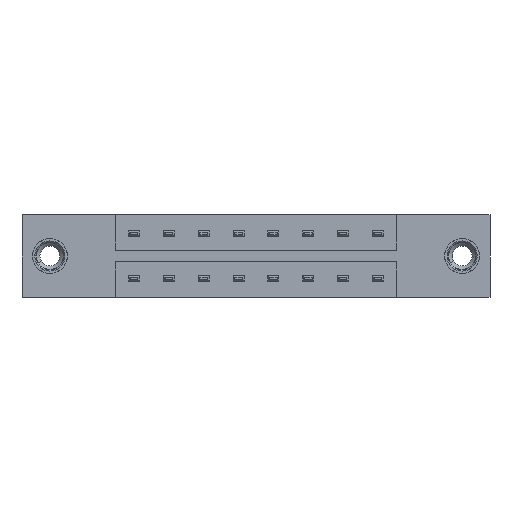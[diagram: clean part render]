
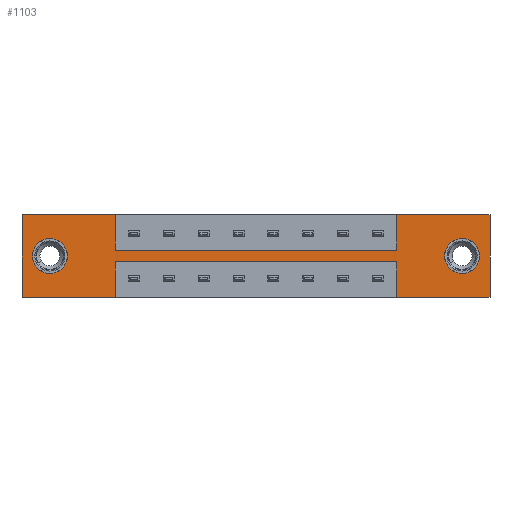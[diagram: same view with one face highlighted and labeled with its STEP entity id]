
A CAD part, front view. The second image highlights one B-rep face of the part: STEP entity #1103.
In plain terms, the highlighted planar face has unit normal (0, -1, 0).
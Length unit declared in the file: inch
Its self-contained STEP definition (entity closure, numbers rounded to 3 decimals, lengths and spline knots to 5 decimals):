
#28 = CARTESIAN_POINT ( 'NONE',  ( 0.125, 0., -0.107 ) ) ;
#279 = CIRCLE ( 'NONE', #1157, 0.078 ) ;
#281 = VERTEX_POINT ( 'NONE', #5145 ) ;
#287 = CARTESIAN_POINT ( 'NONE',  ( 1.6785, 0., -0.2115 ) ) ;
#428 = CARTESIAN_POINT ( 'NONE',  ( 1.971, 0., -0.107 ) ) ;
#557 = ORIENTED_EDGE ( 'NONE', *, *, #6035, .F. ) ;
#691 = FACE_OUTER_BOUND ( 'NONE', #9298, .T. ) ;
#742 = PLANE ( 'NONE',  #9926 ) ;
#753 = CARTESIAN_POINT ( 'NONE',  ( 1.6785, 0., -0.37 ) ) ;
#804 = VECTOR ( 'NONE', #1284, 39.37008 ) ;
#869 = DIRECTION ( 'NONE',  ( 1., 0., 0. ) ) ;
#981 = CARTESIAN_POINT ( 'NONE',  ( 0., 0., 0. ) ) ;
#1083 = ORIENTED_EDGE ( 'NONE', *, *, #9784, .F. ) ;
#1103 = ADVANCED_FACE ( 'NONE', ( #3110, #2244, #691 ), #742, .T. ) ;
#1157 = AXIS2_PLACEMENT_3D ( 'NONE', #9131, #1862, #9195 ) ;
#1270 = DIRECTION ( 'NONE',  ( 0., 0., 1. ) ) ;
#1274 = DIRECTION ( 'NONE',  ( 0., 0., 1. ) ) ;
#1284 = DIRECTION ( 'NONE',  ( -1., 0., 0. ) ) ;
#1367 = CARTESIAN_POINT ( 'NONE',  ( 0., 0., 0. ) ) ;
#1424 = CARTESIAN_POINT ( 'NONE',  ( 1.971, 0., -0.185 ) ) ;
#1503 = VERTEX_POINT ( 'NONE', #9902 ) ;
#1566 = CARTESIAN_POINT ( 'NONE',  ( 2.096, 0., 0. ) ) ;
#1862 = DIRECTION ( 'NONE',  ( 0., 1., 0. ) ) ;
#1921 = EDGE_CURVE ( 'NONE', #9788, #6580, #8120, .T. ) ;
#1945 = LINE ( 'NONE', #7503, #9971 ) ;
#2244 = FACE_BOUND ( 'NONE', #3035, .T. ) ;
#2268 = EDGE_CURVE ( 'NONE', #9918, #7715, #7352, .T. ) ;
#2359 = VECTOR ( 'NONE', #6195, 39.37008 ) ;
#2700 = DIRECTION ( 'NONE',  ( 1., 0., 0. ) ) ;
#2832 = LINE ( 'NONE', #287, #5261 ) ;
#2896 = LINE ( 'NONE', #6126, #8921 ) ;
#2914 = CARTESIAN_POINT ( 'NONE',  ( 0., 0., 0. ) ) ;
#2956 = VERTEX_POINT ( 'NONE', #4046 ) ;
#3035 = EDGE_LOOP ( 'NONE', ( #3039, #9278 ) ) ;
#3039 = ORIENTED_EDGE ( 'NONE', *, *, #2268, .T. ) ;
#3060 = DIRECTION ( 'NONE',  ( 0., 0., 1. ) ) ;
#3110 = FACE_BOUND ( 'NONE', #5142, .T. ) ;
#3137 = DIRECTION ( 'NONE',  ( 0., 1., 0. ) ) ;
#3159 = DIRECTION ( 'NONE',  ( 0., -1., 0. ) ) ;
#3477 = LINE ( 'NONE', #8479, #7918 ) ;
#3536 = DIRECTION ( 'NONE',  ( -1., 0., 0. ) ) ;
#3574 = VECTOR ( 'NONE', #869, 39.37008 ) ;
#3656 = CARTESIAN_POINT ( 'NONE',  ( 1.6785, 0., -0.2115 ) ) ;
#3727 = CARTESIAN_POINT ( 'NONE',  ( 1.6785, 0., 0. ) ) ;
#3862 = CARTESIAN_POINT ( 'NONE',  ( 0.125, 0., -0.185 ) ) ;
#4031 = VERTEX_POINT ( 'NONE', #428 ) ;
#4046 = CARTESIAN_POINT ( 'NONE',  ( 1.6785, 0., -0.1585 ) ) ;
#4050 = EDGE_CURVE ( 'NONE', #4441, #2956, #1945, .T. ) ;
#4241 = CARTESIAN_POINT ( 'NONE',  ( 0.4175, 0., -0.2115 ) ) ;
#4320 = VERTEX_POINT ( 'NONE', #753 ) ;
#4345 = CARTESIAN_POINT ( 'NONE',  ( 0.4175, 0., -0.1585 ) ) ;
#4351 = VERTEX_POINT ( 'NONE', #4241 ) ;
#4441 = VERTEX_POINT ( 'NONE', #4345 ) ;
#4553 = VERTEX_POINT ( 'NONE', #3656 ) ;
#4648 = EDGE_CURVE ( 'NONE', #4553, #4351, #2896, .T. ) ;
#4866 = ORIENTED_EDGE ( 'NONE', *, *, #4648, .F. ) ;
#4871 = CARTESIAN_POINT ( 'NONE',  ( 0.125, 0., -0.263 ) ) ;
#4890 = ORIENTED_EDGE ( 'NONE', *, *, #7141, .T. ) ;
#4947 = CARTESIAN_POINT ( 'NONE',  ( 2.096, 0., 0. ) ) ;
#4978 = EDGE_CURVE ( 'NONE', #2956, #9788, #5379, .T. ) ;
#5051 = DIRECTION ( 'NONE',  ( 0., 0., -1. ) ) ;
#5142 = EDGE_LOOP ( 'NONE', ( #5392, #4890 ) ) ;
#5145 = CARTESIAN_POINT ( 'NONE',  ( 2.096, 0., -0.37 ) ) ;
#5168 = DIRECTION ( 'NONE',  ( 0., 0., -1. ) ) ;
#5187 = LINE ( 'NONE', #5242, #804 ) ;
#5200 = DIRECTION ( 'NONE',  ( 1., 0., 0. ) ) ;
#5224 = ORIENTED_EDGE ( 'NONE', *, *, #7940, .F. ) ;
#5242 = CARTESIAN_POINT ( 'NONE',  ( 0., 0., -0.37 ) ) ;
#5261 = VECTOR ( 'NONE', #1274, 39.37008 ) ;
#5313 = CARTESIAN_POINT ( 'NONE',  ( 0.4175, 0., -0.1585 ) ) ;
#5379 = LINE ( 'NONE', #6961, #9796 ) ;
#5392 = ORIENTED_EDGE ( 'NONE', *, *, #7099, .T. ) ;
#5401 = CIRCLE ( 'NONE', #10505, 0.078 ) ;
#5423 = DIRECTION ( 'NONE',  ( 0., 0., -1. ) ) ;
#5539 = DIRECTION ( 'NONE',  ( 0., 0., -1. ) ) ;
#5666 = AXIS2_PLACEMENT_3D ( 'NONE', #3862, #7077, #3060 ) ;
#5778 = EDGE_CURVE ( 'NONE', #4351, #7856, #7468, .T. ) ;
#5852 = CARTESIAN_POINT ( 'NONE',  ( 0., 0., 0. ) ) ;
#5886 = VECTOR ( 'NONE', #5168, 39.37008 ) ;
#6035 = EDGE_CURVE ( 'NONE', #281, #4320, #3477, .T. ) ;
#6047 = CARTESIAN_POINT ( 'NONE',  ( 0.4175, 0., -0.2115 ) ) ;
#6060 = DIRECTION ( 'NONE',  ( 0., 0., 1. ) ) ;
#6106 = EDGE_CURVE ( 'NONE', #7715, #9918, #5401, .T. ) ;
#6126 = CARTESIAN_POINT ( 'NONE',  ( 0.4175, 0., -0.2115 ) ) ;
#6195 = DIRECTION ( 'NONE',  ( 0., 0., -1. ) ) ;
#6207 = DIRECTION ( 'NONE',  ( 0., 0., 1. ) ) ;
#6260 = CIRCLE ( 'NONE', #7595, 0.078 ) ;
#6570 = ORIENTED_EDGE ( 'NONE', *, *, #4050, .F. ) ;
#6580 = VERTEX_POINT ( 'NONE', #1566 ) ;
#6675 = EDGE_CURVE ( 'NONE', #7856, #1503, #5187, .T. ) ;
#6885 = CARTESIAN_POINT ( 'NONE',  ( 0., 0., -0.37 ) ) ;
#6961 = CARTESIAN_POINT ( 'NONE',  ( 1.6785, 0., -0.1585 ) ) ;
#7077 = DIRECTION ( 'NONE',  ( 0., 1., 0. ) ) ;
#7099 = EDGE_CURVE ( 'NONE', #4031, #7587, #279, .T. ) ;
#7114 = VECTOR ( 'NONE', #5051, 39.37008 ) ;
#7141 = EDGE_CURVE ( 'NONE', #7587, #4031, #6260, .T. ) ;
#7244 = CARTESIAN_POINT ( 'NONE',  ( 1.971, 0., -0.263 ) ) ;
#7352 = CIRCLE ( 'NONE', #5666, 0.078 ) ;
#7468 = LINE ( 'NONE', #6047, #5886 ) ;
#7503 = CARTESIAN_POINT ( 'NONE',  ( 0.4175, 0., -0.1585 ) ) ;
#7511 = ORIENTED_EDGE ( 'NONE', *, *, #8765, .F. ) ;
#7562 = LINE ( 'NONE', #981, #9335 ) ;
#7587 = VERTEX_POINT ( 'NONE', #7244 ) ;
#7595 = AXIS2_PLACEMENT_3D ( 'NONE', #1424, #3137, #5423 ) ;
#7715 = VERTEX_POINT ( 'NONE', #4871 ) ;
#7856 = VERTEX_POINT ( 'NONE', #10258 ) ;
#7918 = VECTOR ( 'NONE', #3536, 39.37008 ) ;
#7927 = EDGE_CURVE ( 'NONE', #6580, #281, #9897, .T. ) ;
#7940 = EDGE_CURVE ( 'NONE', #8412, #9089, #7562, .T. ) ;
#8120 = LINE ( 'NONE', #5852, #3574 ) ;
#8150 = ORIENTED_EDGE ( 'NONE', *, *, #6675, .F. ) ;
#8412 = VERTEX_POINT ( 'NONE', #2914 ) ;
#8479 = CARTESIAN_POINT ( 'NONE',  ( 0., 0., -0.37 ) ) ;
#8683 = ORIENTED_EDGE ( 'NONE', *, *, #7927, .F. ) ;
#8765 = EDGE_CURVE ( 'NONE', #4320, #4553, #2832, .T. ) ;
#8788 = VECTOR ( 'NONE', #6207, 39.37008 ) ;
#8921 = VECTOR ( 'NONE', #9384, 39.37008 ) ;
#9078 = CARTESIAN_POINT ( 'NONE',  ( 0.125, 0., -0.185 ) ) ;
#9089 = VERTEX_POINT ( 'NONE', #9735 ) ;
#9131 = CARTESIAN_POINT ( 'NONE',  ( 1.971, 0., -0.185 ) ) ;
#9195 = DIRECTION ( 'NONE',  ( 0., 0., -1. ) ) ;
#9278 = ORIENTED_EDGE ( 'NONE', *, *, #6106, .T. ) ;
#9290 = EDGE_CURVE ( 'NONE', #1503, #8412, #10433, .T. ) ;
#9298 = EDGE_LOOP ( 'NONE', ( #7511, #557, #8683, #10439, #9566, #6570, #1083, #5224, #9772, #8150, #9624, #4866 ) ) ;
#9335 = VECTOR ( 'NONE', #2700, 39.37008 ) ;
#9384 = DIRECTION ( 'NONE',  ( -1., 0., 0. ) ) ;
#9403 = LINE ( 'NONE', #5313, #2359 ) ;
#9566 = ORIENTED_EDGE ( 'NONE', *, *, #4978, .F. ) ;
#9624 = ORIENTED_EDGE ( 'NONE', *, *, #5778, .F. ) ;
#9735 = CARTESIAN_POINT ( 'NONE',  ( 0.4175, 0., 0. ) ) ;
#9772 = ORIENTED_EDGE ( 'NONE', *, *, #9290, .F. ) ;
#9784 = EDGE_CURVE ( 'NONE', #9089, #4441, #9403, .T. ) ;
#9788 = VERTEX_POINT ( 'NONE', #3727 ) ;
#9796 = VECTOR ( 'NONE', #1270, 39.37008 ) ;
#9897 = LINE ( 'NONE', #4947, #7114 ) ;
#9902 = CARTESIAN_POINT ( 'NONE',  ( 0., 0., -0.37 ) ) ;
#9918 = VERTEX_POINT ( 'NONE', #28 ) ;
#9926 = AXIS2_PLACEMENT_3D ( 'NONE', #6885, #3159, #5539 ) ;
#9971 = VECTOR ( 'NONE', #5200, 39.37008 ) ;
#10078 = DIRECTION ( 'NONE',  ( 0., 1., 0. ) ) ;
#10258 = CARTESIAN_POINT ( 'NONE',  ( 0.4175, 0., -0.37 ) ) ;
#10433 = LINE ( 'NONE', #1367, #8788 ) ;
#10439 = ORIENTED_EDGE ( 'NONE', *, *, #1921, .F. ) ;
#10505 = AXIS2_PLACEMENT_3D ( 'NONE', #9078, #10078, #6060 ) ;
